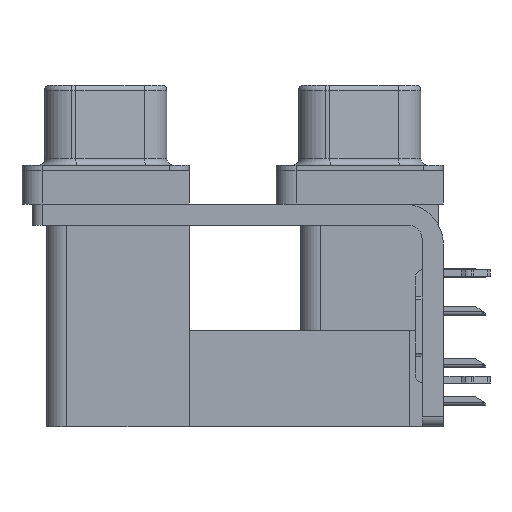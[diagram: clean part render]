
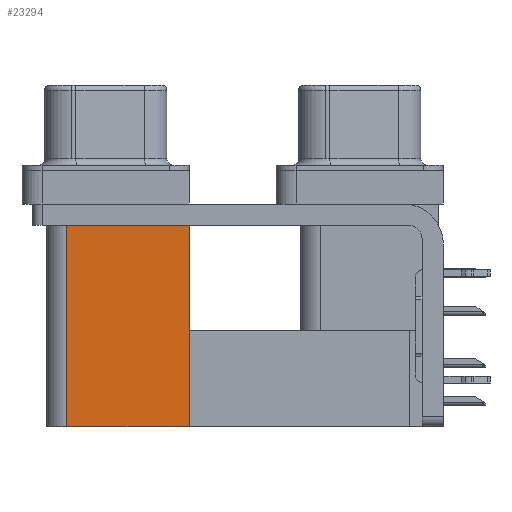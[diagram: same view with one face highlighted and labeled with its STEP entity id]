
A CAD part, left-side view. The second image highlights one B-rep face of the part: STEP entity #23294.
In plain terms, the highlighted planar face has unit normal (-1, 0, 0).
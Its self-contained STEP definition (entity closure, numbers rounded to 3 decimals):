
#298 = ORIENTED_EDGE ( 'NONE', *, *, #13751, .T. ) ;
#374 = VERTEX_POINT ( 'NONE', #21586 ) ;
#428 = DIRECTION ( 'NONE',  ( 0., 1., 0. ) ) ;
#2331 = VERTEX_POINT ( 'NONE', #6453 ) ;
#2851 = LINE ( 'NONE', #18666, #3652 ) ;
#3177 = CARTESIAN_POINT ( 'NONE',  ( 3.765, 12.775, -2.5 ) ) ;
#3652 = VECTOR ( 'NONE', #13518, 1000. ) ;
#6453 = CARTESIAN_POINT ( 'NONE',  ( 3.765, 21.975, -19.2 ) ) ;
#6682 = EDGE_LOOP ( 'NONE', ( #298, #28635, #33876, #28263 ) ) ;
#7330 = CARTESIAN_POINT ( 'NONE',  ( 3.765, 12.775, -19.2 ) ) ;
#9758 = LINE ( 'NONE', #7330, #17846 ) ;
#9786 = EDGE_CURVE ( 'NONE', #374, #2331, #9758, .T. ) ;
#10400 = LINE ( 'NONE', #3177, #11064 ) ;
#10883 = FACE_OUTER_BOUND ( 'NONE', #6682, .T. ) ;
#11064 = VECTOR ( 'NONE', #428, 1000. ) ;
#13518 = DIRECTION ( 'NONE',  ( 0., 0., 1. ) ) ;
#13751 = EDGE_CURVE ( 'NONE', #24273, #20082, #10400, .T. ) ;
#13856 = VECTOR ( 'NONE', #24404, 1000. ) ;
#14698 = CARTESIAN_POINT ( 'NONE',  ( 3.765, 12.775, -2.5 ) ) ;
#15730 = AXIS2_PLACEMENT_3D ( 'NONE', #21754, #32268, #23649 ) ;
#17846 = VECTOR ( 'NONE', #27864, 1000. ) ;
#18666 = CARTESIAN_POINT ( 'NONE',  ( 3.765, 21.975, -19.2 ) ) ;
#20082 = VERTEX_POINT ( 'NONE', #28507 ) ;
#21586 = CARTESIAN_POINT ( 'NONE',  ( 3.765, 12.775, -19.2 ) ) ;
#21754 = CARTESIAN_POINT ( 'NONE',  ( 3.765, 12.775, -19.2 ) ) ;
#22859 = EDGE_CURVE ( 'NONE', #2331, #20082, #2851, .T. ) ;
#23294 = ADVANCED_FACE ( 'NONE', ( #10883 ), #24161, .F. ) ;
#23649 = DIRECTION ( 'NONE',  ( 0., 1., 0. ) ) ;
#24054 = LINE ( 'NONE', #24220, #13856 ) ;
#24161 = PLANE ( 'NONE',  #15730 ) ;
#24220 = CARTESIAN_POINT ( 'NONE',  ( 3.765, 12.775, -19.2 ) ) ;
#24273 = VERTEX_POINT ( 'NONE', #14698 ) ;
#24404 = DIRECTION ( 'NONE',  ( 0., 0., 1. ) ) ;
#27864 = DIRECTION ( 'NONE',  ( 0., 1., 0. ) ) ;
#28263 = ORIENTED_EDGE ( 'NONE', *, *, #32608, .T. ) ;
#28507 = CARTESIAN_POINT ( 'NONE',  ( 3.765, 21.975, -2.5 ) ) ;
#28635 = ORIENTED_EDGE ( 'NONE', *, *, #22859, .F. ) ;
#32268 = DIRECTION ( 'NONE',  ( 1., 0., 0. ) ) ;
#32608 = EDGE_CURVE ( 'NONE', #374, #24273, #24054, .T. ) ;
#33876 = ORIENTED_EDGE ( 'NONE', *, *, #9786, .F. ) ;
